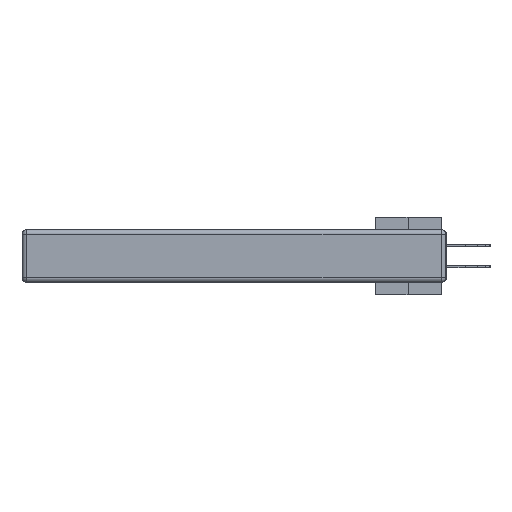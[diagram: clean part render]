
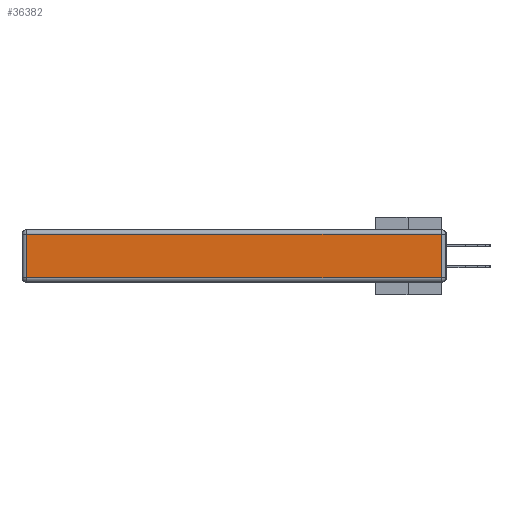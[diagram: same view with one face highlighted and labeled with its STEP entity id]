
A CAD part, left-side view. The second image highlights one B-rep face of the part: STEP entity #36382.
In plain terms, the highlighted planar face has unit normal (-1, 0, 0).
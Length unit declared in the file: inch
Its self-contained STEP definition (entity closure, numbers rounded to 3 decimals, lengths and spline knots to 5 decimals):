
#807 = EDGE_LOOP ( 'NONE', ( #1939, #11348, #5297, #38865 ) ) ;
#1797 = EDGE_CURVE ( 'NONE', #24575, #31247, #38838, .T. ) ;
#1939 = ORIENTED_EDGE ( 'NONE', *, *, #1797, .T. ) ;
#2087 = CARTESIAN_POINT ( 'NONE',  ( 0., 0.03, -0.03 ) ) ;
#3095 = DIRECTION ( 'NONE',  ( 0., 1., 0. ) ) ;
#4316 = DIRECTION ( 'NONE',  ( 0., 0., -1. ) ) ;
#5242 = FACE_OUTER_BOUND ( 'NONE', #807, .T. ) ;
#5297 = ORIENTED_EDGE ( 'NONE', *, *, #6957, .T. ) ;
#5308 = VECTOR ( 'NONE', #37496, 39.37008 ) ;
#5553 = EDGE_CURVE ( 'NONE', #14896, #24575, #36100, .T. ) ;
#5613 = VECTOR ( 'NONE', #3095, 39.37008 ) ;
#6957 = EDGE_CURVE ( 'NONE', #8511, #14896, #40187, .T. ) ;
#7501 = PLANE ( 'NONE',  #7907 ) ;
#7796 = DIRECTION ( 'NONE',  ( -1., 0., 0. ) ) ;
#7907 = AXIS2_PLACEMENT_3D ( 'NONE', #23995, #7796, #13775 ) ;
#8511 = VERTEX_POINT ( 'NONE', #2087 ) ;
#9888 = CARTESIAN_POINT ( 'NONE',  ( 0., 2.75, -0.03 ) ) ;
#11348 = ORIENTED_EDGE ( 'NONE', *, *, #23845, .T. ) ;
#13775 = DIRECTION ( 'NONE',  ( 0., 0., 1. ) ) ;
#14896 = VERTEX_POINT ( 'NONE', #24965 ) ;
#20319 = CARTESIAN_POINT ( 'NONE',  ( 0., 0., -0.313 ) ) ;
#20343 = CARTESIAN_POINT ( 'NONE',  ( 0., 0.03, -0.343 ) ) ;
#23845 = EDGE_CURVE ( 'NONE', #31247, #8511, #27308, .T. ) ;
#23995 = CARTESIAN_POINT ( 'NONE',  ( 0., 0., -0.343 ) ) ;
#24575 = VERTEX_POINT ( 'NONE', #24925 ) ;
#24925 = CARTESIAN_POINT ( 'NONE',  ( 0., 2.72, -0.313 ) ) ;
#24965 = CARTESIAN_POINT ( 'NONE',  ( 0., 2.72, -0.03 ) ) ;
#27308 = LINE ( 'NONE', #20343, #38384 ) ;
#30285 = VECTOR ( 'NONE', #4316, 39.37008 ) ;
#31247 = VERTEX_POINT ( 'NONE', #38890 ) ;
#34410 = CARTESIAN_POINT ( 'NONE',  ( 0., 2.72, -0.343 ) ) ;
#36100 = LINE ( 'NONE', #34410, #30285 ) ;
#36382 = ADVANCED_FACE ( 'NONE', ( #5242 ), #7501, .T. ) ;
#37496 = DIRECTION ( 'NONE',  ( 0., -1., 0. ) ) ;
#38384 = VECTOR ( 'NONE', #39983, 39.37008 ) ;
#38838 = LINE ( 'NONE', #20319, #5308 ) ;
#38865 = ORIENTED_EDGE ( 'NONE', *, *, #5553, .T. ) ;
#38890 = CARTESIAN_POINT ( 'NONE',  ( 0., 0.03, -0.313 ) ) ;
#39983 = DIRECTION ( 'NONE',  ( 0., 0., 1. ) ) ;
#40187 = LINE ( 'NONE', #9888, #5613 ) ;
